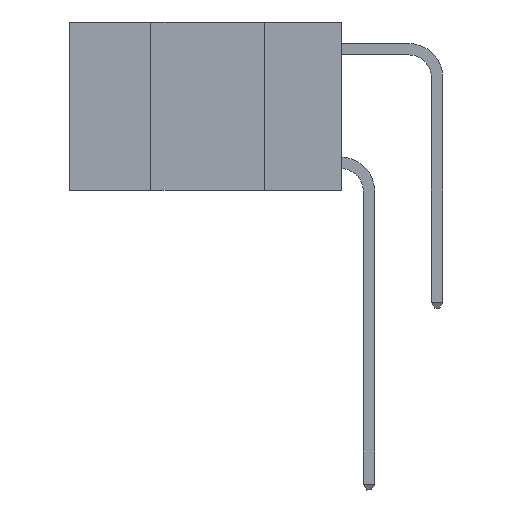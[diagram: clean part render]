
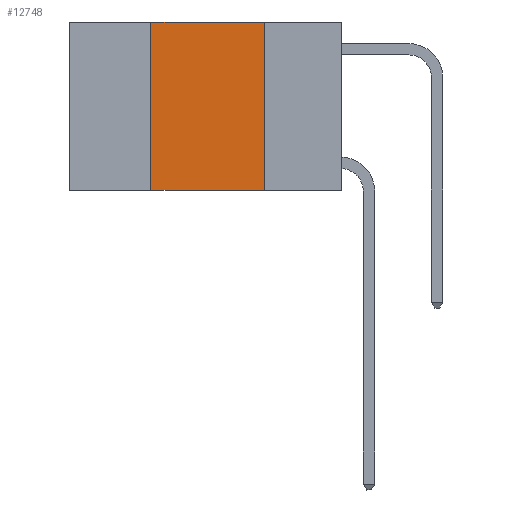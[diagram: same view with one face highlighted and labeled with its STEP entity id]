
A CAD part, left-side view. The second image highlights one B-rep face of the part: STEP entity #12748.
In plain terms, the highlighted planar face has unit normal (-1, 0, 0).
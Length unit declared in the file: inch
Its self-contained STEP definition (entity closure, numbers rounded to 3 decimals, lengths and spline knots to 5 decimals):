
#490 = CARTESIAN_POINT ( 'NONE',  ( 0., 0.17, 0. ) ) ;
#1110 = FACE_OUTER_BOUND ( 'NONE', #16163, .T. ) ;
#1263 = VERTEX_POINT ( 'NONE', #18762 ) ;
#1657 = CARTESIAN_POINT ( 'NONE',  ( 0., 0.42, 0. ) ) ;
#2311 = ORIENTED_EDGE ( 'NONE', *, *, #7668, .F. ) ;
#2442 = ORIENTED_EDGE ( 'NONE', *, *, #14651, .T. ) ;
#3082 = AXIS2_PLACEMENT_3D ( 'NONE', #6486, #18688, #6706 ) ;
#3381 = VERTEX_POINT ( 'NONE', #8099 ) ;
#3697 = CARTESIAN_POINT ( 'NONE',  ( 0., 0.6, -0.37 ) ) ;
#4480 = EDGE_CURVE ( 'NONE', #3381, #1263, #7323, .T. ) ;
#6065 = VECTOR ( 'NONE', #8502, 39.37008 ) ;
#6486 = CARTESIAN_POINT ( 'NONE',  ( 0., 0.6, 0. ) ) ;
#6706 = DIRECTION ( 'NONE',  ( 0., 0., -1. ) ) ;
#7323 = LINE ( 'NONE', #490, #12450 ) ;
#7668 = EDGE_CURVE ( 'NONE', #14724, #3381, #15908, .T. ) ;
#8099 = CARTESIAN_POINT ( 'NONE',  ( 0., 0.17, 0. ) ) ;
#8245 = VECTOR ( 'NONE', #22509, 39.37008 ) ;
#8271 = LINE ( 'NONE', #18538, #19603 ) ;
#8502 = DIRECTION ( 'NONE',  ( 0., -1., 0. ) ) ;
#9015 = ORIENTED_EDGE ( 'NONE', *, *, #4480, .F. ) ;
#9533 = DIRECTION ( 'NONE',  ( 0., 0., 1. ) ) ;
#10442 = CARTESIAN_POINT ( 'NONE',  ( 0., 0.6, 0. ) ) ;
#10548 = VERTEX_POINT ( 'NONE', #12852 ) ;
#10772 = EDGE_CURVE ( 'NONE', #10548, #14724, #8271, .T. ) ;
#12450 = VECTOR ( 'NONE', #21158, 39.37008 ) ;
#12748 = ADVANCED_FACE ( 'NONE', ( #1110 ), #15181, .F. ) ;
#12852 = CARTESIAN_POINT ( 'NONE',  ( 0., 0.42, -0.37 ) ) ;
#12867 = ORIENTED_EDGE ( 'NONE', *, *, #10772, .F. ) ;
#14651 = EDGE_CURVE ( 'NONE', #10548, #1263, #19330, .T. ) ;
#14724 = VERTEX_POINT ( 'NONE', #1657 ) ;
#15181 = PLANE ( 'NONE',  #3082 ) ;
#15908 = LINE ( 'NONE', #10442, #8245 ) ;
#16163 = EDGE_LOOP ( 'NONE', ( #9015, #2311, #12867, #2442 ) ) ;
#18538 = CARTESIAN_POINT ( 'NONE',  ( 0., 0.42, 0. ) ) ;
#18688 = DIRECTION ( 'NONE',  ( 1., 0., 0. ) ) ;
#18762 = CARTESIAN_POINT ( 'NONE',  ( 0., 0.17, -0.37 ) ) ;
#19330 = LINE ( 'NONE', #3697, #6065 ) ;
#19603 = VECTOR ( 'NONE', #9533, 39.37008 ) ;
#21158 = DIRECTION ( 'NONE',  ( 0., 0., -1. ) ) ;
#22509 = DIRECTION ( 'NONE',  ( 0., -1., 0. ) ) ;
